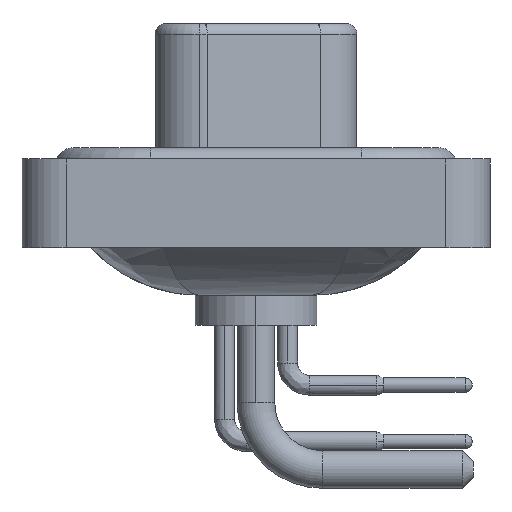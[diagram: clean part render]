
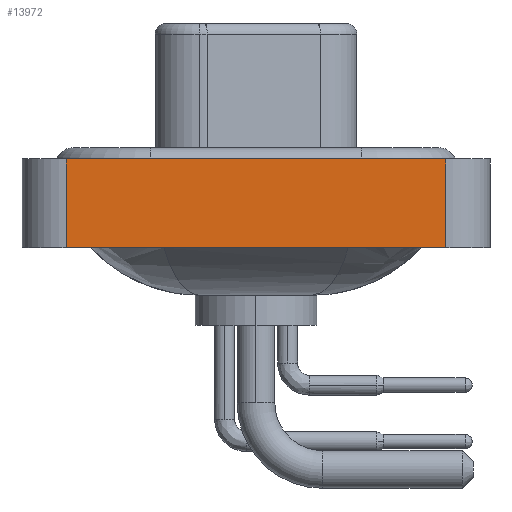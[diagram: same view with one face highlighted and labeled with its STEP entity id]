
A CAD part, left-side view. The second image highlights one B-rep face of the part: STEP entity #13972.
In plain terms, the highlighted planar face has unit normal (-1, 0, 0).
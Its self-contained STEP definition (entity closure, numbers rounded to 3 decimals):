
#805 = EDGE_CURVE ( 'NONE', #10128, #12564, #10408, .T. ) ;
#1118 = LINE ( 'NONE', #9440, #17633 ) ;
#1271 = DIRECTION ( 'NONE',  ( 0., 0., 1. ) ) ;
#1401 = DIRECTION ( 'NONE',  ( -1., 0., 0. ) ) ;
#1504 = DIRECTION ( 'NONE',  ( 0., 0., 1. ) ) ;
#2192 = ORIENTED_EDGE ( 'NONE', *, *, #18806, .T. ) ;
#2630 = LINE ( 'NONE', #24532, #13233 ) ;
#2787 = CARTESIAN_POINT ( 'NONE',  ( -7.35, 8.55, 0.4 ) ) ;
#3384 = CARTESIAN_POINT ( 'NONE',  ( -7.35, -8.55, -3.6 ) ) ;
#4391 = DIRECTION ( 'NONE',  ( 0., -1., 0. ) ) ;
#9440 = CARTESIAN_POINT ( 'NONE',  ( -7.35, -8.55, -3.6 ) ) ;
#10128 = VERTEX_POINT ( 'NONE', #2787 ) ;
#10398 = DIRECTION ( 'NONE',  ( 0., 0., 1. ) ) ;
#10408 = LINE ( 'NONE', #16504, #23868 ) ;
#12187 = EDGE_CURVE ( 'NONE', #22851, #10128, #2630, .T. ) ;
#12564 = VERTEX_POINT ( 'NONE', #14343 ) ;
#12945 = AXIS2_PLACEMENT_3D ( 'NONE', #3384, #1401, #1271 ) ;
#13233 = VECTOR ( 'NONE', #10398, 1000. ) ;
#13972 = ADVANCED_FACE ( 'NONE', ( #21324 ), #21200, .T. ) ;
#14343 = CARTESIAN_POINT ( 'NONE',  ( -7.35, -8.55, 0.4 ) ) ;
#14592 = ORIENTED_EDGE ( 'NONE', *, *, #12187, .F. ) ;
#15437 = VERTEX_POINT ( 'NONE', #17559 ) ;
#16504 = CARTESIAN_POINT ( 'NONE',  ( -7.35, -8.55, 0.4 ) ) ;
#16624 = ORIENTED_EDGE ( 'NONE', *, *, #805, .F. ) ;
#16760 = CARTESIAN_POINT ( 'NONE',  ( -7.35, -8.55, -3.6 ) ) ;
#17559 = CARTESIAN_POINT ( 'NONE',  ( -7.35, -8.55, -3.6 ) ) ;
#17633 = VECTOR ( 'NONE', #1504, 1000. ) ;
#18472 = DIRECTION ( 'NONE',  ( 0., -1., 0. ) ) ;
#18806 = EDGE_CURVE ( 'NONE', #15437, #12564, #1118, .T. ) ;
#19886 = EDGE_CURVE ( 'NONE', #22851, #15437, #24429, .T. ) ;
#21200 = PLANE ( 'NONE',  #12945 ) ;
#21324 = FACE_OUTER_BOUND ( 'NONE', #22527, .T. ) ;
#21917 = VECTOR ( 'NONE', #4391, 1000. ) ;
#22527 = EDGE_LOOP ( 'NONE', ( #2192, #16624, #14592, #22805 ) ) ;
#22805 = ORIENTED_EDGE ( 'NONE', *, *, #19886, .T. ) ;
#22851 = VERTEX_POINT ( 'NONE', #24980 ) ;
#23868 = VECTOR ( 'NONE', #18472, 1000. ) ;
#24429 = LINE ( 'NONE', #16760, #21917 ) ;
#24532 = CARTESIAN_POINT ( 'NONE',  ( -7.35, 8.55, -3.6 ) ) ;
#24980 = CARTESIAN_POINT ( 'NONE',  ( -7.35, 8.55, -3.6 ) ) ;
